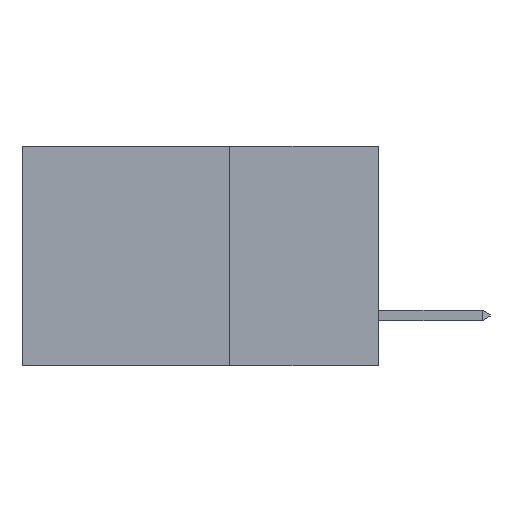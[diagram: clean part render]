
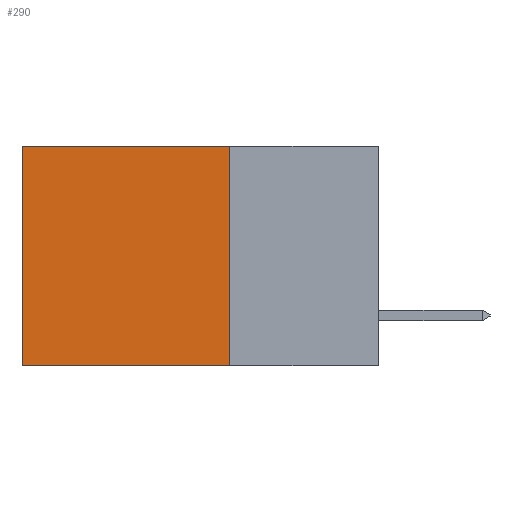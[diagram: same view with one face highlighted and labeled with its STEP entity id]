
A CAD part, left-side view. The second image highlights one B-rep face of the part: STEP entity #290.
In plain terms, the highlighted planar face has unit normal (-1, 0, 0).
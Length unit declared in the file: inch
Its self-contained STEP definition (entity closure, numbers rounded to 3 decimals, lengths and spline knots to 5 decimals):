
#290 = ADVANCED_FACE ( 'NONE', ( #315 ), #1864, .F. ) ;
#315 = FACE_OUTER_BOUND ( 'NONE', #4577, .T. ) ;
#399 = VECTOR ( 'NONE', #6603, 39.37008 ) ;
#844 = VERTEX_POINT ( 'NONE', #8432 ) ;
#864 = LINE ( 'NONE', #2385, #399 ) ;
#1162 = CARTESIAN_POINT ( 'NONE',  ( 0.298, 0.25, 0. ) ) ;
#1541 = ORIENTED_EDGE ( 'NONE', *, *, #7801, .F. ) ;
#1560 = CARTESIAN_POINT ( 'NONE',  ( 0.298, 0.6, 0. ) ) ;
#1718 = EDGE_CURVE ( 'NONE', #5567, #6406, #864, .T. ) ;
#1832 = DIRECTION ( 'NONE',  ( 0., 0., -1. ) ) ;
#1864 = PLANE ( 'NONE',  #3136 ) ;
#1924 = DIRECTION ( 'NONE',  ( 0., 1., 0. ) ) ;
#2141 = VECTOR ( 'NONE', #1924, 39.37008 ) ;
#2385 = CARTESIAN_POINT ( 'NONE',  ( 0.298, 0.25, 0. ) ) ;
#3029 = ORIENTED_EDGE ( 'NONE', *, *, #1718, .F. ) ;
#3136 = AXIS2_PLACEMENT_3D ( 'NONE', #8289, #7323, #7341 ) ;
#3681 = LINE ( 'NONE', #8096, #9610 ) ;
#4378 = LINE ( 'NONE', #1162, #2141 ) ;
#4577 = EDGE_LOOP ( 'NONE', ( #8107, #1541, #3029, #4785 ) ) ;
#4785 = ORIENTED_EDGE ( 'NONE', *, *, #8173, .T. ) ;
#4791 = LINE ( 'NONE', #1560, #6841 ) ;
#5567 = VERTEX_POINT ( 'NONE', #6730 ) ;
#5845 = CARTESIAN_POINT ( 'NONE',  ( 0.298, 0.25, -0.37 ) ) ;
#6054 = CARTESIAN_POINT ( 'NONE',  ( 0.298, 0.6, 0. ) ) ;
#6406 = VERTEX_POINT ( 'NONE', #5845 ) ;
#6578 = EDGE_CURVE ( 'NONE', #6816, #844, #4791, .T. ) ;
#6603 = DIRECTION ( 'NONE',  ( 0., 0., -1. ) ) ;
#6730 = CARTESIAN_POINT ( 'NONE',  ( 0.298, 0.25, 0. ) ) ;
#6816 = VERTEX_POINT ( 'NONE', #6054 ) ;
#6841 = VECTOR ( 'NONE', #1832, 39.37008 ) ;
#7323 = DIRECTION ( 'NONE',  ( 1., 0., 0. ) ) ;
#7341 = DIRECTION ( 'NONE',  ( 0., 0., -1. ) ) ;
#7357 = DIRECTION ( 'NONE',  ( 0., 1., 0. ) ) ;
#7801 = EDGE_CURVE ( 'NONE', #6406, #844, #3681, .T. ) ;
#8096 = CARTESIAN_POINT ( 'NONE',  ( 0.298, 0.25, -0.37 ) ) ;
#8107 = ORIENTED_EDGE ( 'NONE', *, *, #6578, .T. ) ;
#8173 = EDGE_CURVE ( 'NONE', #5567, #6816, #4378, .T. ) ;
#8289 = CARTESIAN_POINT ( 'NONE',  ( 0.298, 0.25, 0. ) ) ;
#8432 = CARTESIAN_POINT ( 'NONE',  ( 0.298, 0.6, -0.37 ) ) ;
#9610 = VECTOR ( 'NONE', #7357, 39.37008 ) ;
